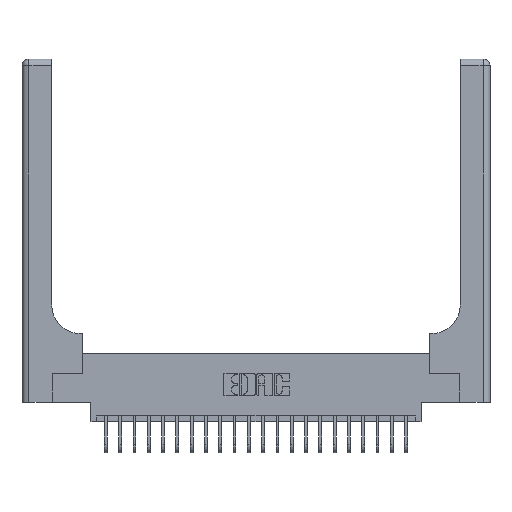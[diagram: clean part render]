
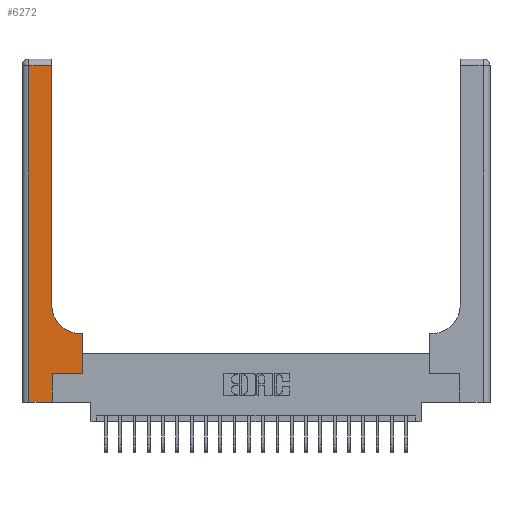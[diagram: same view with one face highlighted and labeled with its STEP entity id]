
A CAD part, top view. The second image highlights one B-rep face of the part: STEP entity #6272.
In plain terms, the highlighted planar face has unit normal (0, 0, 1).
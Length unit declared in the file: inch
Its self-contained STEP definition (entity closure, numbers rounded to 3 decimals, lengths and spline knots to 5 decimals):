
#58 = AXIS2_PLACEMENT_3D ( 'NONE', #3280, #18369, #10650 ) ;
#317 = ORIENTED_EDGE ( 'NONE', *, *, #22350, .T. ) ;
#1212 = VERTEX_POINT ( 'NONE', #21281 ) ;
#1347 = LINE ( 'NONE', #9749, #9520 ) ;
#3280 = CARTESIAN_POINT ( 'NONE',  ( 0., 3., 0.37 ) ) ;
#3339 = VECTOR ( 'NONE', #11275, 39.37008 ) ;
#3366 = ORIENTED_EDGE ( 'NONE', *, *, #4990, .T. ) ;
#4422 = DIRECTION ( 'NONE',  ( 0., 1., 0. ) ) ;
#4990 = EDGE_CURVE ( 'NONE', #23341, #10678, #9533, .T. ) ;
#5128 = CARTESIAN_POINT ( 'NONE',  ( 0.528, 0.25, 0.37 ) ) ;
#5301 = CARTESIAN_POINT ( 'NONE',  ( 0., 2.94, 0.37 ) ) ;
#5397 = LINE ( 'NONE', #18596, #19709 ) ;
#6219 = AXIS2_PLACEMENT_3D ( 'NONE', #21388, #23256, #15663 ) ;
#6272 = ADVANCED_FACE ( 'NONE', ( #17092 ), #12661, .F. ) ;
#6345 = CARTESIAN_POINT ( 'NONE',  ( 0.06, 3., 0.37 ) ) ;
#6585 = ORIENTED_EDGE ( 'NONE', *, *, #20583, .T. ) ;
#7174 = DIRECTION ( 'NONE',  ( -1., 0., 0. ) ) ;
#7326 = CARTESIAN_POINT ( 'NONE',  ( 0.26, 2.94, 0.37 ) ) ;
#8843 = EDGE_CURVE ( 'NONE', #10678, #21469, #1347, .T. ) ;
#9278 = CARTESIAN_POINT ( 'NONE',  ( 0.528, 0.6, 0.37 ) ) ;
#9458 = DIRECTION ( 'NONE',  ( 1., 0., 0. ) ) ;
#9520 = VECTOR ( 'NONE', #21545, 39.37008 ) ;
#9533 = LINE ( 'NONE', #14389, #13315 ) ;
#9631 = ORIENTED_EDGE ( 'NONE', *, *, #9756, .T. ) ;
#9749 = CARTESIAN_POINT ( 'NONE',  ( 0.265, 0., 0.37 ) ) ;
#9756 = EDGE_CURVE ( 'NONE', #21469, #18619, #5397, .T. ) ;
#9790 = VERTEX_POINT ( 'NONE', #16756 ) ;
#10222 = EDGE_CURVE ( 'NONE', #20981, #1212, #14678, .T. ) ;
#10650 = DIRECTION ( 'NONE',  ( -1., 0., 0. ) ) ;
#10653 = VECTOR ( 'NONE', #7174, 39.37008 ) ;
#10678 = VERTEX_POINT ( 'NONE', #20188 ) ;
#11043 = CARTESIAN_POINT ( 'NONE',  ( 0.26, 0.6, 0.37 ) ) ;
#11275 = DIRECTION ( 'NONE',  ( -1., 0., 0. ) ) ;
#11439 = EDGE_CURVE ( 'NONE', #18619, #23839, #18770, .T. ) ;
#11515 = VECTOR ( 'NONE', #13507, 39.37008 ) ;
#11666 = LINE ( 'NONE', #20834, #22177 ) ;
#12372 = VECTOR ( 'NONE', #4422, 39.37008 ) ;
#12391 = LINE ( 'NONE', #6345, #11515 ) ;
#12661 = PLANE ( 'NONE',  #58 ) ;
#12986 = CARTESIAN_POINT ( 'NONE',  ( 0.51, 0.6, 0.37 ) ) ;
#13315 = VECTOR ( 'NONE', #23851, 39.37008 ) ;
#13507 = DIRECTION ( 'NONE',  ( 0., -1., 0. ) ) ;
#13575 = EDGE_CURVE ( 'NONE', #9790, #20981, #11666, .T. ) ;
#14081 = VERTEX_POINT ( 'NONE', #12986 ) ;
#14389 = CARTESIAN_POINT ( 'NONE',  ( 0., 0., 0.37 ) ) ;
#14422 = LINE ( 'NONE', #11043, #3339 ) ;
#14678 = LINE ( 'NONE', #5301, #10653 ) ;
#15663 = DIRECTION ( 'NONE',  ( 1., 0., 0. ) ) ;
#15805 = ORIENTED_EDGE ( 'NONE', *, *, #18856, .T. ) ;
#16036 = ORIENTED_EDGE ( 'NONE', *, *, #8843, .T. ) ;
#16383 = EDGE_LOOP ( 'NONE', ( #17872, #23988, #317, #3366, #16036, #9631, #16558, #15805, #6585 ) ) ;
#16558 = ORIENTED_EDGE ( 'NONE', *, *, #11439, .T. ) ;
#16756 = CARTESIAN_POINT ( 'NONE',  ( 0.26, 0.85, 0.37 ) ) ;
#17092 = FACE_OUTER_BOUND ( 'NONE', #16383, .T. ) ;
#17152 = CARTESIAN_POINT ( 'NONE',  ( 0.528, 0.25, 0.37 ) ) ;
#17872 = ORIENTED_EDGE ( 'NONE', *, *, #13575, .T. ) ;
#18369 = DIRECTION ( 'NONE',  ( 0., 0., -1. ) ) ;
#18596 = CARTESIAN_POINT ( 'NONE',  ( 0.265, 0.25, 0.37 ) ) ;
#18619 = VERTEX_POINT ( 'NONE', #5128 ) ;
#18770 = LINE ( 'NONE', #17152, #12372 ) ;
#18856 = EDGE_CURVE ( 'NONE', #23839, #14081, #14422, .T. ) ;
#18881 = DIRECTION ( 'NONE',  ( 0., 1., 0. ) ) ;
#19322 = CIRCLE ( 'NONE', #6219, 0.25 ) ;
#19709 = VECTOR ( 'NONE', #9458, 39.37008 ) ;
#19801 = CARTESIAN_POINT ( 'NONE',  ( 0.265, 0.25, 0.37 ) ) ;
#20188 = CARTESIAN_POINT ( 'NONE',  ( 0.265, 0., 0.37 ) ) ;
#20242 = CARTESIAN_POINT ( 'NONE',  ( 0.06, 0., 0.37 ) ) ;
#20583 = EDGE_CURVE ( 'NONE', #14081, #9790, #19322, .T. ) ;
#20834 = CARTESIAN_POINT ( 'NONE',  ( 0.26, 3., 0.37 ) ) ;
#20981 = VERTEX_POINT ( 'NONE', #7326 ) ;
#21281 = CARTESIAN_POINT ( 'NONE',  ( 0.06, 2.94, 0.37 ) ) ;
#21388 = CARTESIAN_POINT ( 'NONE',  ( 0.51, 0.85, 0.37 ) ) ;
#21469 = VERTEX_POINT ( 'NONE', #19801 ) ;
#21545 = DIRECTION ( 'NONE',  ( 0., 1., 0. ) ) ;
#22177 = VECTOR ( 'NONE', #18881, 39.37008 ) ;
#22350 = EDGE_CURVE ( 'NONE', #1212, #23341, #12391, .T. ) ;
#23256 = DIRECTION ( 'NONE',  ( 0., 0., -1. ) ) ;
#23341 = VERTEX_POINT ( 'NONE', #20242 ) ;
#23839 = VERTEX_POINT ( 'NONE', #9278 ) ;
#23851 = DIRECTION ( 'NONE',  ( 1., 0., 0. ) ) ;
#23988 = ORIENTED_EDGE ( 'NONE', *, *, #10222, .T. ) ;
